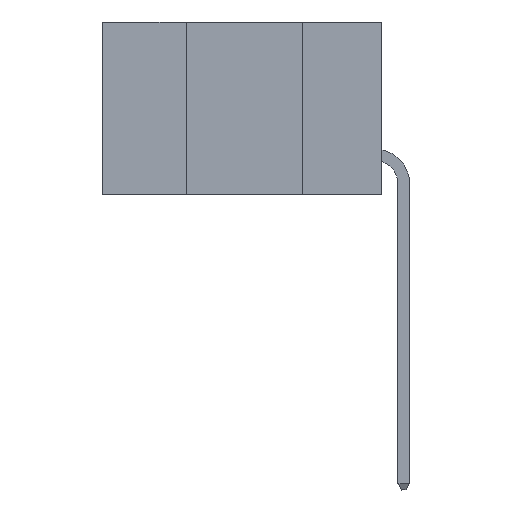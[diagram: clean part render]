
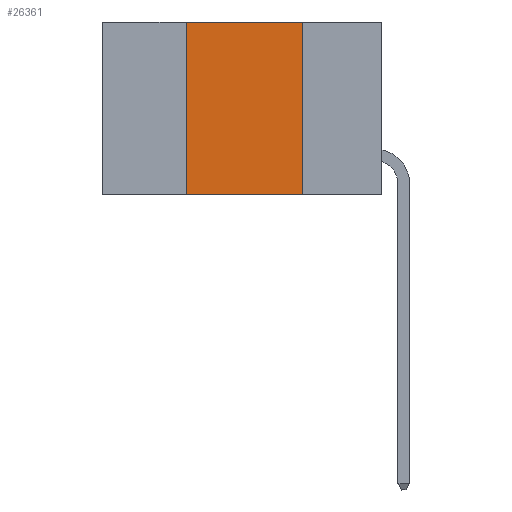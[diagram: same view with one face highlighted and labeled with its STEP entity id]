
A CAD part, left-side view. The second image highlights one B-rep face of the part: STEP entity #26361.
In plain terms, the highlighted planar face has unit normal (-1, 0, 0).
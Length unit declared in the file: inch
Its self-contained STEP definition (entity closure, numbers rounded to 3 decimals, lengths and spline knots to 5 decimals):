
#19 = DIRECTION ( 'NONE',  ( 1., 0., 0. ) ) ;
#2326 = CARTESIAN_POINT ( 'NONE',  ( 0., 0.17, 0. ) ) ;
#2780 = EDGE_LOOP ( 'NONE', ( #6256, #36611, #43137, #42933 ) ) ;
#5149 = VECTOR ( 'NONE', #18350, 39.37008 ) ;
#6256 = ORIENTED_EDGE ( 'NONE', *, *, #46423, .F. ) ;
#9307 = CARTESIAN_POINT ( 'NONE',  ( 0., 0.42, 0. ) ) ;
#9473 = VECTOR ( 'NONE', #32966, 39.37008 ) ;
#11695 = DIRECTION ( 'NONE',  ( 0., 0., -1. ) ) ;
#12731 = AXIS2_PLACEMENT_3D ( 'NONE', #23815, #19, #11695 ) ;
#16377 = CARTESIAN_POINT ( 'NONE',  ( 0., 0.42, -0.37 ) ) ;
#18350 = DIRECTION ( 'NONE',  ( 0., -1., 0. ) ) ;
#22667 = CARTESIAN_POINT ( 'NONE',  ( 0., 0.6, -0.37 ) ) ;
#23815 = CARTESIAN_POINT ( 'NONE',  ( 0., 0.6, 0. ) ) ;
#24441 = VERTEX_POINT ( 'NONE', #33422 ) ;
#24588 = DIRECTION ( 'NONE',  ( 0., 0., 1. ) ) ;
#25673 = EDGE_CURVE ( 'NONE', #34796, #31823, #49215, .T. ) ;
#26361 = ADVANCED_FACE ( 'NONE', ( #31763 ), #39996, .F. ) ;
#27189 = VECTOR ( 'NONE', #24588, 39.37008 ) ;
#28037 = VECTOR ( 'NONE', #43039, 39.37008 ) ;
#30409 = EDGE_CURVE ( 'NONE', #39870, #24441, #32555, .T. ) ;
#31763 = FACE_OUTER_BOUND ( 'NONE', #2780, .T. ) ;
#31823 = VERTEX_POINT ( 'NONE', #2326 ) ;
#32555 = LINE ( 'NONE', #22667, #5149 ) ;
#32966 = DIRECTION ( 'NONE',  ( 0., 0., -1. ) ) ;
#33422 = CARTESIAN_POINT ( 'NONE',  ( 0., 0.17, -0.37 ) ) ;
#34796 = VERTEX_POINT ( 'NONE', #36599 ) ;
#36599 = CARTESIAN_POINT ( 'NONE',  ( 0., 0.42, 0. ) ) ;
#36611 = ORIENTED_EDGE ( 'NONE', *, *, #25673, .F. ) ;
#36963 = CARTESIAN_POINT ( 'NONE',  ( 0., 0.17, 0. ) ) ;
#39300 = EDGE_CURVE ( 'NONE', #39870, #34796, #41483, .T. ) ;
#39870 = VERTEX_POINT ( 'NONE', #16377 ) ;
#39996 = PLANE ( 'NONE',  #12731 ) ;
#41483 = LINE ( 'NONE', #9307, #27189 ) ;
#42933 = ORIENTED_EDGE ( 'NONE', *, *, #30409, .T. ) ;
#43039 = DIRECTION ( 'NONE',  ( 0., -1., 0. ) ) ;
#43137 = ORIENTED_EDGE ( 'NONE', *, *, #39300, .F. ) ;
#46423 = EDGE_CURVE ( 'NONE', #31823, #24441, #49288, .T. ) ;
#49215 = LINE ( 'NONE', #51556, #28037 ) ;
#49288 = LINE ( 'NONE', #36963, #9473 ) ;
#51556 = CARTESIAN_POINT ( 'NONE',  ( 0., 0.6, 0. ) ) ;
